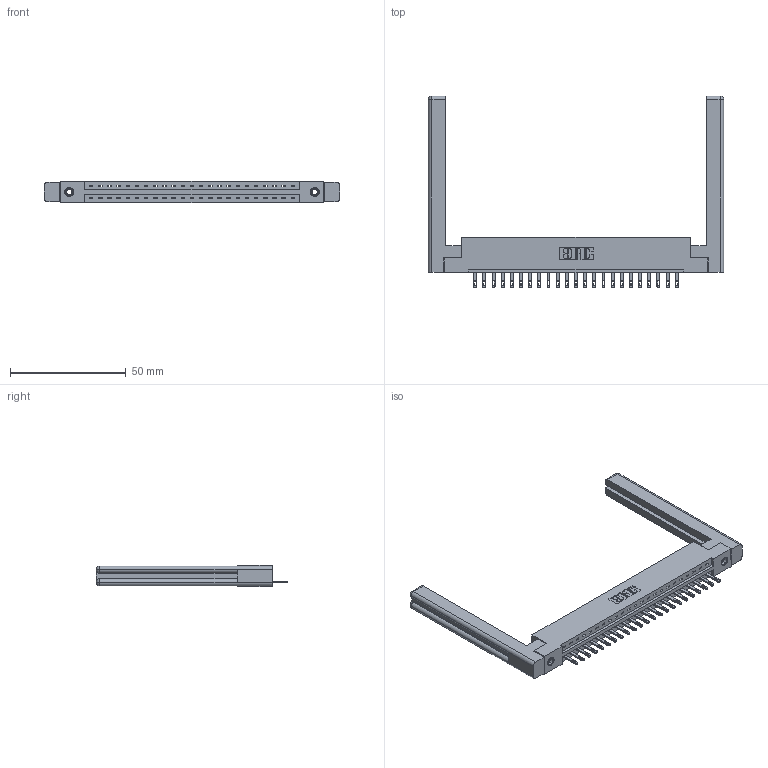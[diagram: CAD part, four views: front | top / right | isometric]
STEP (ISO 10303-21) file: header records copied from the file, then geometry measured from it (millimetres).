
FILE_DESCRIPTION (( 'STEP AP203' ), '1' );
FILE_NAME ('337-023-500-158.STEP', '2019-09-30T14:12:17', ( '' ), ( '' ), 'SwSTEP 2.0', 'SolidWorks 2016', '' );
FILE_SCHEMA (( 'CONFIG_CONTROL_DESIGN' ));
Length unit declared in the file: inch
Products named in the file (5): 337-023-500-158; 307-220-058; 337 Part_Flush Mounting Lugs - 0.156 Dia-TI; 345-292-001_345-293-100; 345-250-001_345-250-001-102
Assembly tree (28 placements, depth 2):
  337-023-500-158
    337 Part_Flush Mounting Lugs - 0.156 Dia-TI
    345-292-001_345-293-100  x23
    345-250-001_345-250-001-102  x2
    307-220-058  x2
Bounding box: 127.76 x 82.94 x 9.4 mm (x, y, z)
Volume: 20217.3 mm3; surface area: 18651.9 mm2
Topology: 28 solids, 28 shells, 1590 faces, 4805 edges, 3190 vertices
Faces by surface type: plane 1074, cylinder 492, cone 12, torus 12
Entity records: 22118 total; most frequent: CARTESIAN_POINT 3850, ORIENTED_EDGE 3748, DIRECTION 3300, EDGE_CURVE 1874, LINE 1694, VECTOR 1694, VERTEX_POINT 1242, AXIS2_PLACEMENT_3D 803
